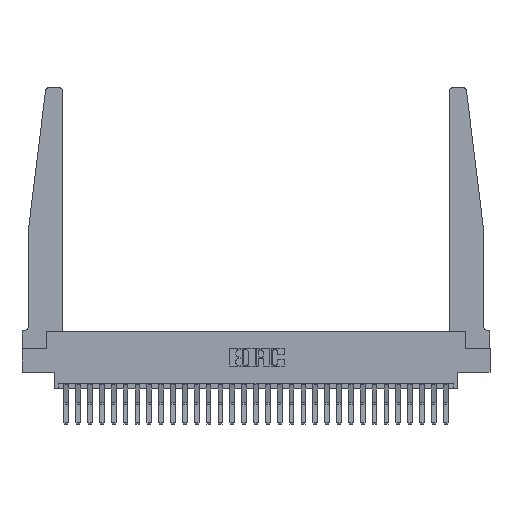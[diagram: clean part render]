
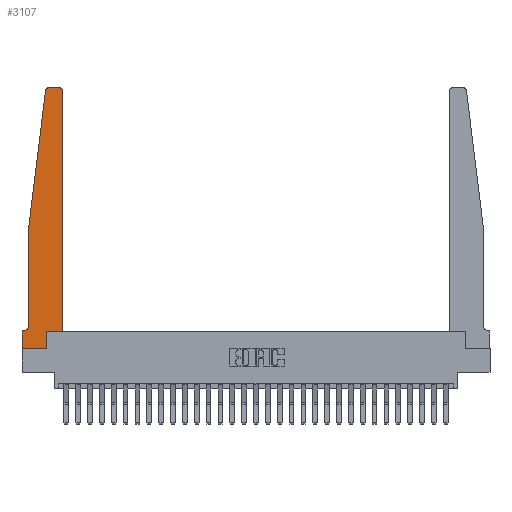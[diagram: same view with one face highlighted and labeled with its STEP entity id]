
A CAD part, top view. The second image highlights one B-rep face of the part: STEP entity #3107.
In plain terms, the highlighted planar face has unit normal (0, 0, 1).
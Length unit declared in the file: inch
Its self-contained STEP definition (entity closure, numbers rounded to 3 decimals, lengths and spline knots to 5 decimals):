
#56 = CARTESIAN_POINT ( 'NONE',  ( 0.065, 1.25, 0.37 ) ) ;
#370 = VERTEX_POINT ( 'NONE', #22147 ) ;
#566 = EDGE_CURVE ( 'NONE', #13826, #1807, #17361, .T. ) ;
#1133 = VECTOR ( 'NONE', #23518, 39.37008 ) ;
#1807 = VERTEX_POINT ( 'NONE', #15208 ) ;
#2077 = ORIENTED_EDGE ( 'NONE', *, *, #23296, .T. ) ;
#2087 = EDGE_CURVE ( 'NONE', #8963, #23045, #26008, .T. ) ;
#2452 = EDGE_CURVE ( 'NONE', #22240, #5414, #17274, .T. ) ;
#2936 = CARTESIAN_POINT ( 'NONE',  ( 0., 0., 0.37 ) ) ;
#3107 = ADVANCED_FACE ( 'NONE', ( #11844 ), #25047, .T. ) ;
#3529 = CARTESIAN_POINT ( 'NONE',  ( 0.065, 0.1875, 0.37 ) ) ;
#4105 = CIRCLE ( 'NONE', #17282, 0.03 ) ;
#4158 = CARTESIAN_POINT ( 'NONE',  ( 0.395, 2.75, 0.37 ) ) ;
#4336 = VERTEX_POINT ( 'NONE', #4158 ) ;
#4746 = CARTESIAN_POINT ( 'NONE',  ( 0.015, 0.1875, 0.37 ) ) ;
#4946 = CIRCLE ( 'NONE', #11312, 0.03 ) ;
#5305 = EDGE_CURVE ( 'NONE', #1807, #4336, #4946, .T. ) ;
#5414 = VERTEX_POINT ( 'NONE', #10201 ) ;
#5644 = ORIENTED_EDGE ( 'NONE', *, *, #2087, .T. ) ;
#6887 = DIRECTION ( 'NONE',  ( -1., 0., 0. ) ) ;
#6928 = DIRECTION ( 'NONE',  ( 1., 0., 0. ) ) ;
#7596 = EDGE_CURVE ( 'NONE', #24926, #22240, #4105, .T. ) ;
#8215 = DIRECTION ( 'NONE',  ( -1., 0., 0. ) ) ;
#8334 = EDGE_CURVE ( 'NONE', #23045, #13826, #17742, .T. ) ;
#8425 = DIRECTION ( 'NONE',  ( 0., 1., 0. ) ) ;
#8493 = LINE ( 'NONE', #3529, #19027 ) ;
#8555 = VECTOR ( 'NONE', #24782, 39.37008 ) ;
#8862 = DIRECTION ( 'NONE',  ( 1., 0., 0. ) ) ;
#8963 = VERTEX_POINT ( 'NONE', #18095 ) ;
#8965 = CARTESIAN_POINT ( 'NONE',  ( 0.2605, 0.18, 0.37 ) ) ;
#9174 = DIRECTION ( 'NONE',  ( 0., 0., 1. ) ) ;
#10183 = VECTOR ( 'NONE', #21885, 39.37008 ) ;
#10201 = CARTESIAN_POINT ( 'NONE',  ( 0.065, 1.25, 0.37 ) ) ;
#11003 = CARTESIAN_POINT ( 'NONE',  ( 0.27653, 2.72, 0.37 ) ) ;
#11010 = ORIENTED_EDGE ( 'NONE', *, *, #23378, .T. ) ;
#11237 = CARTESIAN_POINT ( 'NONE',  ( 0.065, 0.2375, 0.37 ) ) ;
#11312 = AXIS2_PLACEMENT_3D ( 'NONE', #19771, #9174, #6928 ) ;
#11844 = FACE_OUTER_BOUND ( 'NONE', #20228, .T. ) ;
#11902 = CARTESIAN_POINT ( 'NONE',  ( 0.24675, 2.72367, 0.37 ) ) ;
#12029 = DIRECTION ( 'NONE',  ( 0., -1., 0. ) ) ;
#12168 = EDGE_CURVE ( 'NONE', #14874, #13428, #24317, .T. ) ;
#12667 = DIRECTION ( 'NONE',  ( 0., 1., 0. ) ) ;
#13428 = VERTEX_POINT ( 'NONE', #4746 ) ;
#13826 = VERTEX_POINT ( 'NONE', #20111 ) ;
#14217 = AXIS2_PLACEMENT_3D ( 'NONE', #20596, #18422, #27188 ) ;
#14874 = VERTEX_POINT ( 'NONE', #11237 ) ;
#15208 = CARTESIAN_POINT ( 'NONE',  ( 0.425, 2.72, 0.37 ) ) ;
#15470 = EDGE_CURVE ( 'NONE', #4336, #24926, #20621, .T. ) ;
#16317 = CARTESIAN_POINT ( 'NONE',  ( 0., 0., 0.37 ) ) ;
#16392 = VECTOR ( 'NONE', #23937, 39.37008 ) ;
#16769 = ORIENTED_EDGE ( 'NONE', *, *, #8334, .T. ) ;
#16796 = CARTESIAN_POINT ( 'NONE',  ( 0.425, 0.18, 0.37 ) ) ;
#17274 = LINE ( 'NONE', #56, #10183 ) ;
#17282 = AXIS2_PLACEMENT_3D ( 'NONE', #11003, #19714, #8862 ) ;
#17361 = LINE ( 'NONE', #16796, #21526 ) ;
#17742 = LINE ( 'NONE', #24482, #16392 ) ;
#18095 = CARTESIAN_POINT ( 'NONE',  ( 0.2605, 0., 0.37 ) ) ;
#18162 = LINE ( 'NONE', #2936, #22713 ) ;
#18227 = ORIENTED_EDGE ( 'NONE', *, *, #12168, .T. ) ;
#18422 = DIRECTION ( 'NONE',  ( 0., 0., 1. ) ) ;
#18641 = ORIENTED_EDGE ( 'NONE', *, *, #7596, .T. ) ;
#18677 = CARTESIAN_POINT ( 'NONE',  ( 0.2605, 0.18, 0.37 ) ) ;
#19027 = VECTOR ( 'NONE', #8215, 39.37008 ) ;
#19092 = CARTESIAN_POINT ( 'NONE',  ( 0.27653, 2.75, 0.37 ) ) ;
#19645 = EDGE_CURVE ( 'NONE', #370, #8963, #22943, .T. ) ;
#19714 = DIRECTION ( 'NONE',  ( 0., 0., 1. ) ) ;
#19771 = CARTESIAN_POINT ( 'NONE',  ( 0.395, 2.72, 0.37 ) ) ;
#20111 = CARTESIAN_POINT ( 'NONE',  ( 0.425, 0.18, 0.37 ) ) ;
#20228 = EDGE_LOOP ( 'NONE', ( #26099, #18641, #21138, #11010, #18227, #20854, #2077, #20975, #5644, #16769, #22060, #26172 ) ) ;
#20340 = LINE ( 'NONE', #27222, #8555 ) ;
#20596 = CARTESIAN_POINT ( 'NONE',  ( 0., 0.1875, 0.37 ) ) ;
#20621 = LINE ( 'NONE', #23218, #26641 ) ;
#20854 = ORIENTED_EDGE ( 'NONE', *, *, #27733, .T. ) ;
#20975 = ORIENTED_EDGE ( 'NONE', *, *, #19645, .T. ) ;
#21138 = ORIENTED_EDGE ( 'NONE', *, *, #2452, .T. ) ;
#21526 = VECTOR ( 'NONE', #12667, 39.37008 ) ;
#21761 = VERTEX_POINT ( 'NONE', #23909 ) ;
#21885 = DIRECTION ( 'NONE',  ( -0.122, -0.992, 0. ) ) ;
#22035 = CARTESIAN_POINT ( 'NONE',  ( 0.015, 0.2375, 0.37 ) ) ;
#22060 = ORIENTED_EDGE ( 'NONE', *, *, #566, .T. ) ;
#22147 = CARTESIAN_POINT ( 'NONE',  ( 0., 0., 0.37 ) ) ;
#22174 = DIRECTION ( 'NONE',  ( 0., 0., -1. ) ) ;
#22240 = VERTEX_POINT ( 'NONE', #11902 ) ;
#22464 = AXIS2_PLACEMENT_3D ( 'NONE', #22035, #22174, #6887 ) ;
#22495 = VECTOR ( 'NONE', #8425, 39.37008 ) ;
#22713 = VECTOR ( 'NONE', #12029, 39.37008 ) ;
#22943 = LINE ( 'NONE', #16317, #1133 ) ;
#23045 = VERTEX_POINT ( 'NONE', #18677 ) ;
#23218 = CARTESIAN_POINT ( 'NONE',  ( 0.25, 2.75, 0.37 ) ) ;
#23296 = EDGE_CURVE ( 'NONE', #21761, #370, #18162, .T. ) ;
#23378 = EDGE_CURVE ( 'NONE', #5414, #14874, #20340, .T. ) ;
#23518 = DIRECTION ( 'NONE',  ( 1., 0., 0. ) ) ;
#23909 = CARTESIAN_POINT ( 'NONE',  ( 0., 0.1875, 0.37 ) ) ;
#23937 = DIRECTION ( 'NONE',  ( 1., 0., 0. ) ) ;
#24317 = CIRCLE ( 'NONE', #22464, 0.05 ) ;
#24482 = CARTESIAN_POINT ( 'NONE',  ( 0.425, 0.18, 0.37 ) ) ;
#24782 = DIRECTION ( 'NONE',  ( 0., -1., 0. ) ) ;
#24926 = VERTEX_POINT ( 'NONE', #19092 ) ;
#25047 = PLANE ( 'NONE',  #14217 ) ;
#25220 = DIRECTION ( 'NONE',  ( -1., 0., 0. ) ) ;
#26008 = LINE ( 'NONE', #8965, #22495 ) ;
#26099 = ORIENTED_EDGE ( 'NONE', *, *, #15470, .T. ) ;
#26172 = ORIENTED_EDGE ( 'NONE', *, *, #5305, .T. ) ;
#26641 = VECTOR ( 'NONE', #25220, 39.37008 ) ;
#27188 = DIRECTION ( 'NONE',  ( 1., 0., 0. ) ) ;
#27222 = CARTESIAN_POINT ( 'NONE',  ( 0.065, 1.25, 0.37 ) ) ;
#27733 = EDGE_CURVE ( 'NONE', #13428, #21761, #8493, .T. ) ;
